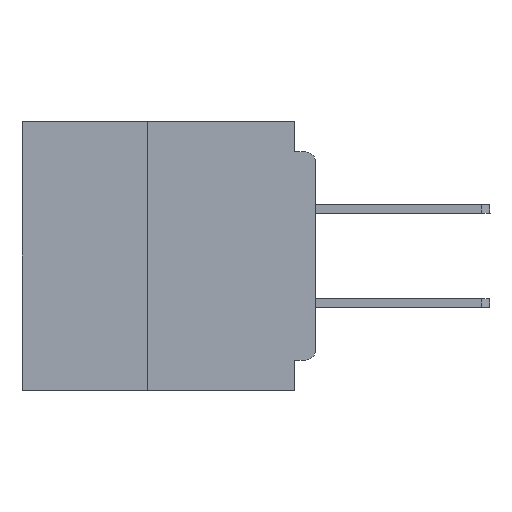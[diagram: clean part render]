
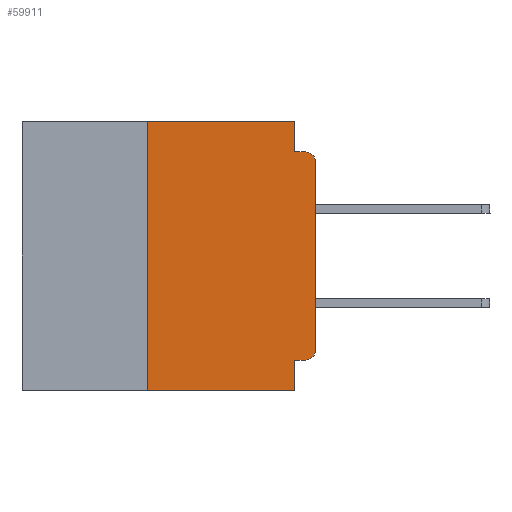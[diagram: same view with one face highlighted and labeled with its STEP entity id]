
A CAD part, left-side view. The second image highlights one B-rep face of the part: STEP entity #59911.
In plain terms, the highlighted planar face has unit normal (-1, 0, 0).
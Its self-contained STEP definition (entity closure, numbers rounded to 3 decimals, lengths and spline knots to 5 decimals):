
#331 = VECTOR ( 'NONE', #41500, 39.37008 ) ;
#438 = EDGE_CURVE ( 'NONE', #45681, #8248, #43021, .T. ) ;
#464 = VERTEX_POINT ( 'NONE', #43700 ) ;
#1758 = VECTOR ( 'NONE', #25073, 39.37008 ) ;
#3026 = VECTOR ( 'NONE', #60294, 39.37008 ) ;
#3158 = ORIENTED_EDGE ( 'NONE', *, *, #44152, .T. ) ;
#3343 = VECTOR ( 'NONE', #12637, 39.37008 ) ;
#3746 = DIRECTION ( 'NONE',  ( 0., 0., 1. ) ) ;
#3847 = DIRECTION ( 'NONE',  ( 1., 0., 0. ) ) ;
#4306 = ORIENTED_EDGE ( 'NONE', *, *, #37087, .F. ) ;
#4649 = LINE ( 'NONE', #34970, #3026 ) ;
#4876 = VECTOR ( 'NONE', #3746, 39.37008 ) ;
#6979 = DIRECTION ( 'NONE',  ( -1., 0., 0. ) ) ;
#8085 = ORIENTED_EDGE ( 'NONE', *, *, #54237, .F. ) ;
#8248 = VERTEX_POINT ( 'NONE', #21683 ) ;
#10321 = AXIS2_PLACEMENT_3D ( 'NONE', #59912, #29392, #64985 ) ;
#10378 = VERTEX_POINT ( 'NONE', #34919 ) ;
#11931 = VERTEX_POINT ( 'NONE', #47892 ) ;
#12268 = ORIENTED_EDGE ( 'NONE', *, *, #14172, .T. ) ;
#12637 = DIRECTION ( 'NONE',  ( 0., -1., 0. ) ) ;
#13988 = CARTESIAN_POINT ( 'NONE',  ( 0., 0., 0. ) ) ;
#14172 = EDGE_CURVE ( 'NONE', #464, #25782, #54437, .T. ) ;
#14215 = VECTOR ( 'NONE', #28233, 39.37008 ) ;
#14237 = CARTESIAN_POINT ( 'NONE',  ( 0., 0.25, 0. ) ) ;
#14593 = CARTESIAN_POINT ( 'NONE',  ( 0., 0.031, 0. ) ) ;
#15749 = CARTESIAN_POINT ( 'NONE',  ( 0., 0., -0.045 ) ) ;
#16485 = CARTESIAN_POINT ( 'NONE',  ( 0., 0., -0.06 ) ) ;
#16958 = FACE_OUTER_BOUND ( 'NONE', #33514, .T. ) ;
#17194 = EDGE_CURVE ( 'NONE', #32034, #10378, #65864, .T. ) ;
#17834 = ORIENTED_EDGE ( 'NONE', *, *, #42183, .T. ) ;
#18698 = ORIENTED_EDGE ( 'NONE', *, *, #36896, .F. ) ;
#20160 = ORIENTED_EDGE ( 'NONE', *, *, #48301, .T. ) ;
#21683 = CARTESIAN_POINT ( 'NONE',  ( 0., 0.031, -0.355 ) ) ;
#21763 = AXIS2_PLACEMENT_3D ( 'NONE', #37548, #6979, #42692 ) ;
#22032 = VERTEX_POINT ( 'NONE', #57410 ) ;
#25073 = DIRECTION ( 'NONE',  ( 0., -1., 0. ) ) ;
#25782 = VERTEX_POINT ( 'NONE', #60778 ) ;
#28233 = DIRECTION ( 'NONE',  ( 0., 1., 0. ) ) ;
#29077 = LINE ( 'NONE', #15749, #331 ) ;
#29392 = DIRECTION ( 'NONE',  ( -1., 0., 0. ) ) ;
#31034 = ORIENTED_EDGE ( 'NONE', *, *, #17194, .F. ) ;
#32034 = VERTEX_POINT ( 'NONE', #14593 ) ;
#32925 = CARTESIAN_POINT ( 'NONE',  ( 0., 0.25, -0.4 ) ) ;
#33514 = EDGE_LOOP ( 'NONE', ( #3158, #20160, #18698, #31034, #8085, #4306, #12268, #39923, #54605, #17834 ) ) ;
#34429 = CARTESIAN_POINT ( 'NONE',  ( 0., 0.437, 0. ) ) ;
#34665 = EDGE_CURVE ( 'NONE', #8248, #25782, #4649, .T. ) ;
#34919 = CARTESIAN_POINT ( 'NONE',  ( 0., 0.031, -0.045 ) ) ;
#34970 = CARTESIAN_POINT ( 'NONE',  ( 0., 0.031, -0.4 ) ) ;
#35419 = CARTESIAN_POINT ( 'NONE',  ( 0., 0.437, -0.4 ) ) ;
#35604 = VERTEX_POINT ( 'NONE', #16485 ) ;
#36896 = EDGE_CURVE ( 'NONE', #10378, #22032, #29077, .T. ) ;
#37052 = CARTESIAN_POINT ( 'NONE',  ( 0., 0.031, 0. ) ) ;
#37087 = EDGE_CURVE ( 'NONE', #464, #55667, #41902, .T. ) ;
#37548 = CARTESIAN_POINT ( 'NONE',  ( 0., 0.015, -0.06 ) ) ;
#38911 = VECTOR ( 'NONE', #47335, 39.37008 ) ;
#39596 = DIRECTION ( 'NONE',  ( 0., 0., -1. ) ) ;
#39923 = ORIENTED_EDGE ( 'NONE', *, *, #34665, .F. ) ;
#40873 = AXIS2_PLACEMENT_3D ( 'NONE', #34429, #3847, #39596 ) ;
#41500 = DIRECTION ( 'NONE',  ( 0., -1., 0. ) ) ;
#41902 = LINE ( 'NONE', #32925, #43494 ) ;
#42183 = EDGE_CURVE ( 'NONE', #45681, #11931, #53160, .T. ) ;
#42692 = DIRECTION ( 'NONE',  ( 0., 0., -1. ) ) ;
#43021 = LINE ( 'NONE', #63846, #14215 ) ;
#43494 = VECTOR ( 'NONE', #63400, 39.37008 ) ;
#43700 = CARTESIAN_POINT ( 'NONE',  ( 0., 0.25, -0.4 ) ) ;
#44029 = LINE ( 'NONE', #13988, #4876 ) ;
#44152 = EDGE_CURVE ( 'NONE', #11931, #35604, #44029, .T. ) ;
#45681 = VERTEX_POINT ( 'NONE', #55085 ) ;
#47335 = DIRECTION ( 'NONE',  ( 0., 0., -1. ) ) ;
#47892 = CARTESIAN_POINT ( 'NONE',  ( 0., 0., -0.34 ) ) ;
#48301 = EDGE_CURVE ( 'NONE', #35604, #22032, #57414, .T. ) ;
#53160 = CIRCLE ( 'NONE', #10321, 0.015 ) ;
#54237 = EDGE_CURVE ( 'NONE', #55667, #32034, #57571, .T. ) ;
#54437 = LINE ( 'NONE', #35419, #1758 ) ;
#54605 = ORIENTED_EDGE ( 'NONE', *, *, #438, .F. ) ;
#55085 = CARTESIAN_POINT ( 'NONE',  ( 0., 0.015, -0.355 ) ) ;
#55667 = VERTEX_POINT ( 'NONE', #14237 ) ;
#57410 = CARTESIAN_POINT ( 'NONE',  ( 0., 0.015, -0.045 ) ) ;
#57414 = CIRCLE ( 'NONE', #21763, 0.015 ) ;
#57571 = LINE ( 'NONE', #58546, #3343 ) ;
#58546 = CARTESIAN_POINT ( 'NONE',  ( 0., 0.437, 0. ) ) ;
#59769 = PLANE ( 'NONE',  #40873 ) ;
#59911 = ADVANCED_FACE ( 'NONE', ( #16958 ), #59769, .F. ) ;
#59912 = CARTESIAN_POINT ( 'NONE',  ( 0., 0.015, -0.34 ) ) ;
#60294 = DIRECTION ( 'NONE',  ( 0., 0., -1. ) ) ;
#60778 = CARTESIAN_POINT ( 'NONE',  ( 0., 0.031, -0.4 ) ) ;
#63400 = DIRECTION ( 'NONE',  ( 0., 0., 1. ) ) ;
#63846 = CARTESIAN_POINT ( 'NONE',  ( 0., 0., -0.355 ) ) ;
#64985 = DIRECTION ( 'NONE',  ( 0., 0., -1. ) ) ;
#65864 = LINE ( 'NONE', #37052, #38911 ) ;
